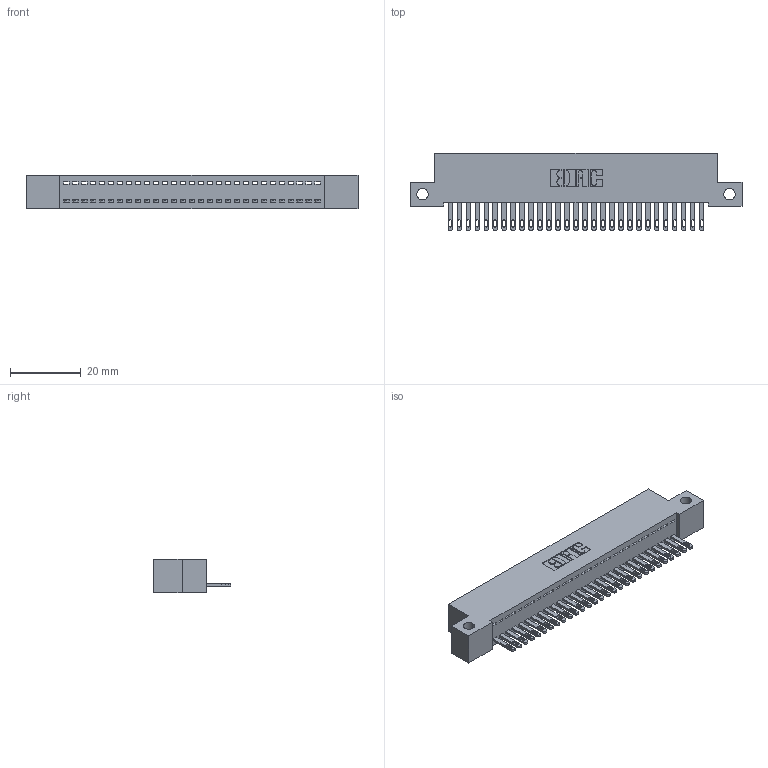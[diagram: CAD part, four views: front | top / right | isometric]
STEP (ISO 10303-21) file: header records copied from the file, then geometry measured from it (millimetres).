
FILE_DESCRIPTION (( 'STEP AP203' ), '1' );
FILE_NAME ('892-029-500-112.STEP', '2020-09-21T15:02:56', ( '' ), ( '' ), 'SwSTEP 2.0', 'SolidWorks 2020', '' );
FILE_SCHEMA (( 'CONFIG_CONTROL_DESIGN' ));
Length unit declared in the file: inch
Products named in the file (3): 345-292-001_345-293-100; 842 Part_Side Mount; 892-029-500-112
Assembly tree (30 placements, depth 2):
  892-029-500-112
    842 Part_Side Mount
    345-292-001_345-293-100  x29
Bounding box: 93.98 x 21.85 x 9.4 mm (x, y, z)
Volume: 8136.3 mm3; surface area: 11599.1 mm2
Topology: 30 solids, 30 shells, 1676 faces, 5171 edges, 3446 vertices
Faces by surface type: plane 1110, cylinder 566
Entity records: 19211 total; most frequent: CARTESIAN_POINT 3321, ORIENTED_EDGE 3286, DIRECTION 2829, EDGE_CURVE 1643, VECTOR 1511, LINE 1511, VERTEX_POINT 1094, AXIS2_PLACEMENT_3D 659
